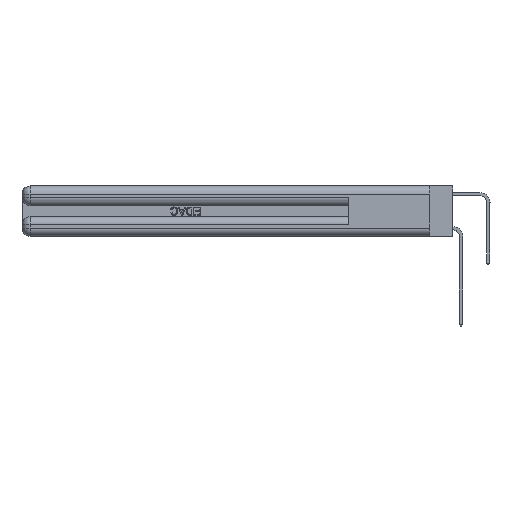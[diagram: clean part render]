
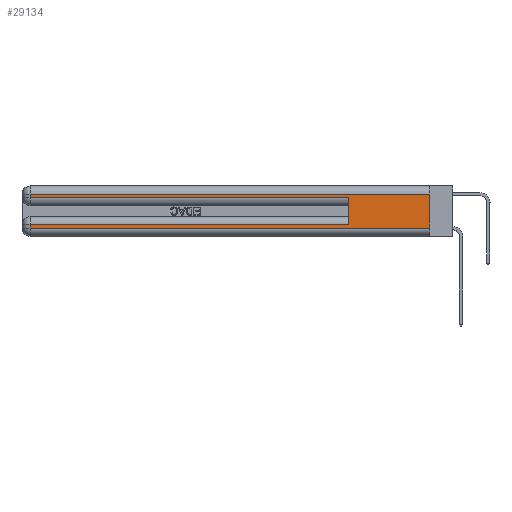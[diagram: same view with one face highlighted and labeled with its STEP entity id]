
A CAD part, left-side view. The second image highlights one B-rep face of the part: STEP entity #29134.
In plain terms, the highlighted planar face has unit normal (-1, 0, 0).
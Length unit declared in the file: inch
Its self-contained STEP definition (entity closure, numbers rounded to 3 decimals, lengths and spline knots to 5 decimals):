
#1473 = ORIENTED_EDGE ( 'NONE', *, *, #13736, .T. ) ;
#2486 = EDGE_CURVE ( 'NONE', #24115, #25518, #7499, .T. ) ;
#3131 = CARTESIAN_POINT ( 'NONE',  ( 0., 2.94, 0.06 ) ) ;
#3422 = EDGE_CURVE ( 'NONE', #31947, #25518, #12692, .T. ) ;
#3977 = CARTESIAN_POINT ( 'NONE',  ( 0., 0., 0.31 ) ) ;
#4453 = DIRECTION ( 'NONE',  ( 0., 0., -1. ) ) ;
#4754 = VECTOR ( 'NONE', #7546, 39.37008 ) ;
#5660 = VECTOR ( 'NONE', #26785, 39.37008 ) ;
#6436 = EDGE_CURVE ( 'NONE', #9375, #31947, #12516, .T. ) ;
#6697 = LINE ( 'NONE', #11765, #24224 ) ;
#6798 = LINE ( 'NONE', #34482, #14708 ) ;
#7499 = LINE ( 'NONE', #31164, #13707 ) ;
#7546 = DIRECTION ( 'NONE',  ( 0., 0., 1. ) ) ;
#7940 = EDGE_CURVE ( 'NONE', #14393, #24460, #29195, .T. ) ;
#8073 = VECTOR ( 'NONE', #25109, 39.37008 ) ;
#8244 = VERTEX_POINT ( 'NONE', #18561 ) ;
#8662 = AXIS2_PLACEMENT_3D ( 'NONE', #33715, #12110, #4453 ) ;
#9375 = VERTEX_POINT ( 'NONE', #13988 ) ;
#9537 = ORIENTED_EDGE ( 'NONE', *, *, #7940, .T. ) ;
#9869 = ORIENTED_EDGE ( 'NONE', *, *, #22692, .F. ) ;
#11449 = VERTEX_POINT ( 'NONE', #25022 ) ;
#11765 = CARTESIAN_POINT ( 'NONE',  ( 0., 0., 0.085 ) ) ;
#12110 = DIRECTION ( 'NONE',  ( 1., 0., 0. ) ) ;
#12516 = LINE ( 'NONE', #17960, #33001 ) ;
#12692 = LINE ( 'NONE', #32010, #5660 ) ;
#12820 = DIRECTION ( 'NONE',  ( 0., 0., -1. ) ) ;
#13086 = DIRECTION ( 'NONE',  ( 0., 1., 0. ) ) ;
#13485 = FACE_OUTER_BOUND ( 'NONE', #15885, .T. ) ;
#13707 = VECTOR ( 'NONE', #23202, 39.37008 ) ;
#13736 = EDGE_CURVE ( 'NONE', #8244, #9375, #6697, .T. ) ;
#13988 = CARTESIAN_POINT ( 'NONE',  ( 0., 2.94, 0.085 ) ) ;
#14393 = VERTEX_POINT ( 'NONE', #19687 ) ;
#14708 = VECTOR ( 'NONE', #13086, 39.37008 ) ;
#15037 = PLANE ( 'NONE',  #8662 ) ;
#15885 = EDGE_LOOP ( 'NONE', ( #27881, #34192, #19695, #9537, #9869, #1473, #29305, #21070 ) ) ;
#17960 = CARTESIAN_POINT ( 'NONE',  ( 0., 2.94, 0.37 ) ) ;
#18561 = CARTESIAN_POINT ( 'NONE',  ( 0., 0.6, 0.085 ) ) ;
#18904 = LINE ( 'NONE', #23505, #4754 ) ;
#19687 = CARTESIAN_POINT ( 'NONE',  ( 0., 2.94, 0.285 ) ) ;
#19695 = ORIENTED_EDGE ( 'NONE', *, *, #23093, .T. ) ;
#20032 = DIRECTION ( 'NONE',  ( 0., 1., 0. ) ) ;
#21070 = ORIENTED_EDGE ( 'NONE', *, *, #3422, .T. ) ;
#22692 = EDGE_CURVE ( 'NONE', #8244, #24460, #18904, .T. ) ;
#22743 = EDGE_CURVE ( 'NONE', #24115, #11449, #6798, .T. ) ;
#23093 = EDGE_CURVE ( 'NONE', #11449, #14393, #31903, .T. ) ;
#23202 = DIRECTION ( 'NONE',  ( 0., 0., -1. ) ) ;
#23505 = CARTESIAN_POINT ( 'NONE',  ( 0., 0.6, 0.145 ) ) ;
#24115 = VERTEX_POINT ( 'NONE', #3977 ) ;
#24224 = VECTOR ( 'NONE', #20032, 39.37008 ) ;
#24460 = VERTEX_POINT ( 'NONE', #29729 ) ;
#25022 = CARTESIAN_POINT ( 'NONE',  ( 0., 2.94, 0.31 ) ) ;
#25109 = DIRECTION ( 'NONE',  ( 0., 0., -1. ) ) ;
#25468 = CARTESIAN_POINT ( 'NONE',  ( 0., 2.94, 0.37 ) ) ;
#25518 = VERTEX_POINT ( 'NONE', #25648 ) ;
#25648 = CARTESIAN_POINT ( 'NONE',  ( 0., 0., 0.06 ) ) ;
#26686 = VECTOR ( 'NONE', #30384, 39.37008 ) ;
#26785 = DIRECTION ( 'NONE',  ( 0., -1., 0. ) ) ;
#27881 = ORIENTED_EDGE ( 'NONE', *, *, #2486, .F. ) ;
#28089 = CARTESIAN_POINT ( 'NONE',  ( 0., 0., 0.285 ) ) ;
#29134 = ADVANCED_FACE ( 'NONE', ( #13485 ), #15037, .F. ) ;
#29195 = LINE ( 'NONE', #28089, #26686 ) ;
#29305 = ORIENTED_EDGE ( 'NONE', *, *, #6436, .T. ) ;
#29729 = CARTESIAN_POINT ( 'NONE',  ( 0., 0.6, 0.285 ) ) ;
#30384 = DIRECTION ( 'NONE',  ( 0., -1., 0. ) ) ;
#31164 = CARTESIAN_POINT ( 'NONE',  ( 0., 0., 0.37 ) ) ;
#31903 = LINE ( 'NONE', #25468, #8073 ) ;
#31947 = VERTEX_POINT ( 'NONE', #3131 ) ;
#32010 = CARTESIAN_POINT ( 'NONE',  ( 0., 0., 0.06 ) ) ;
#33001 = VECTOR ( 'NONE', #12820, 39.37008 ) ;
#33715 = CARTESIAN_POINT ( 'NONE',  ( 0., 0., 0.37 ) ) ;
#34192 = ORIENTED_EDGE ( 'NONE', *, *, #22743, .T. ) ;
#34482 = CARTESIAN_POINT ( 'NONE',  ( 0., 0., 0.31 ) ) ;
